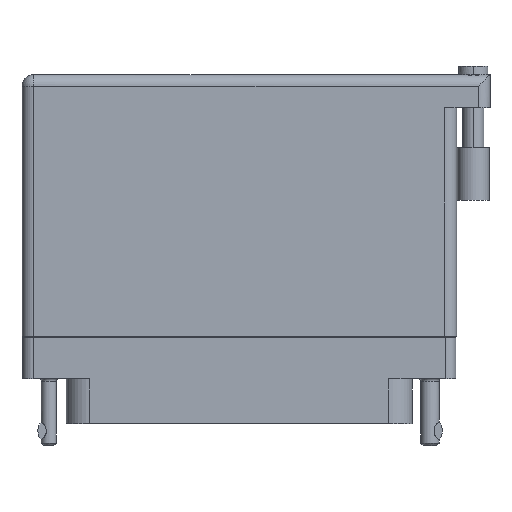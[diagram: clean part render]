
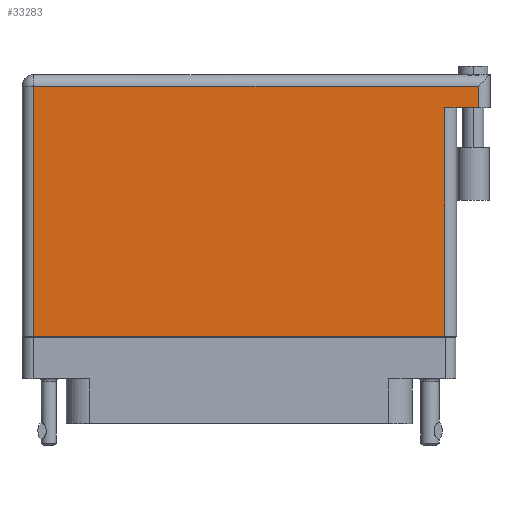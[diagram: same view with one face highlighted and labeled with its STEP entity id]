
A CAD part, front view. The second image highlights one B-rep face of the part: STEP entity #33283.
In plain terms, the highlighted face is planar.
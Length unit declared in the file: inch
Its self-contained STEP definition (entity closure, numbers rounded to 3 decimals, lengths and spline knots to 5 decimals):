
#1376 = CARTESIAN_POINT ( 'NONE',  ( 1.5, 1.269, 0.4495 ) ) ;
#2505 = LINE ( 'NONE', #43728, #18639 ) ;
#3583 = EDGE_CURVE ( 'NONE', #32225, #38675, #10501, .T. ) ;
#4847 = VECTOR ( 'NONE', #8271, 39.37008 ) ;
#5888 = ORIENTED_EDGE ( 'NONE', *, *, #9104, .T. ) ;
#6386 = CARTESIAN_POINT ( 'NONE',  ( 1.43, 1.466, 0.4495 ) ) ;
#7424 = ORIENTED_EDGE ( 'NONE', *, *, #3583, .T. ) ;
#8132 = DIRECTION ( 'NONE',  ( -1., 0., 0. ) ) ;
#8271 = DIRECTION ( 'NONE',  ( 0., -1., 0. ) ) ;
#8437 = PLANE ( 'NONE',  #33535 ) ;
#9104 = EDGE_CURVE ( 'NONE', #41778, #9441, #37307, .T. ) ;
#9441 = VERTEX_POINT ( 'NONE', #53388 ) ;
#10501 = LINE ( 'NONE', #29242, #32436 ) ;
#13491 = CARTESIAN_POINT ( 'NONE',  ( 1.23, 1.269, 0.4495 ) ) ;
#13547 = VERTEX_POINT ( 'NONE', #25972 ) ;
#13910 = CARTESIAN_POINT ( 'NONE',  ( -1.3, 1.396, 0.4495 ) ) ;
#14077 = VECTOR ( 'NONE', #29746, 39.37008 ) ;
#15924 = LINE ( 'NONE', #6386, #14077 ) ;
#18639 = VECTOR ( 'NONE', #25286, 39.37008 ) ;
#24770 = LINE ( 'NONE', #1376, #42360 ) ;
#25286 = DIRECTION ( 'NONE',  ( 1., 0., 0. ) ) ;
#25972 = CARTESIAN_POINT ( 'NONE',  ( 1.43, 1.269, 0.4495 ) ) ;
#27483 = FACE_OUTER_BOUND ( 'NONE', #33182, .T. ) ;
#29242 = CARTESIAN_POINT ( 'NONE',  ( 1.23, 1.269, 0.4495 ) ) ;
#29746 = DIRECTION ( 'NONE',  ( 0., 1., 0. ) ) ;
#30366 = CARTESIAN_POINT ( 'NONE',  ( 1.43, 1.396, 0.4495 ) ) ;
#31012 = EDGE_CURVE ( 'NONE', #9441, #52813, #31626, .T. ) ;
#31626 = LINE ( 'NONE', #50403, #4847 ) ;
#32225 = VERTEX_POINT ( 'NONE', #48055 ) ;
#32436 = VECTOR ( 'NONE', #56341, 39.37008 ) ;
#33182 = EDGE_LOOP ( 'NONE', ( #41082, #7424, #33226, #47063, #5888, #39187 ) ) ;
#33226 = ORIENTED_EDGE ( 'NONE', *, *, #40800, .F. ) ;
#33283 = ADVANCED_FACE ( 'NONE', ( #27483 ), #8437, .F. ) ;
#33535 = AXIS2_PLACEMENT_3D ( 'NONE', #36129, #54859, #8132 ) ;
#36129 = CARTESIAN_POINT ( 'NONE',  ( -1.3, 1.466, 0.4495 ) ) ;
#37307 = LINE ( 'NONE', #13910, #59516 ) ;
#38675 = VERTEX_POINT ( 'NONE', #13491 ) ;
#39187 = ORIENTED_EDGE ( 'NONE', *, *, #31012, .T. ) ;
#40800 = EDGE_CURVE ( 'NONE', #13547, #38675, #24770, .T. ) ;
#41082 = ORIENTED_EDGE ( 'NONE', *, *, #55887, .T. ) ;
#41778 = VERTEX_POINT ( 'NONE', #30366 ) ;
#42360 = VECTOR ( 'NONE', #43808, 39.37008 ) ;
#42504 = DIRECTION ( 'NONE',  ( -1., 0., 0. ) ) ;
#43728 = CARTESIAN_POINT ( 'NONE',  ( -1.3, -0.1, 0.4495 ) ) ;
#43808 = DIRECTION ( 'NONE',  ( -1., 0., 0. ) ) ;
#44584 = EDGE_CURVE ( 'NONE', #13547, #41778, #15924, .T. ) ;
#47063 = ORIENTED_EDGE ( 'NONE', *, *, #44584, .T. ) ;
#48055 = CARTESIAN_POINT ( 'NONE',  ( 1.23, -0.1, 0.4495 ) ) ;
#50403 = CARTESIAN_POINT ( 'NONE',  ( -1.23, -0.1, 0.4495 ) ) ;
#52813 = VERTEX_POINT ( 'NONE', #54882 ) ;
#53388 = CARTESIAN_POINT ( 'NONE',  ( -1.23, 1.396, 0.4495 ) ) ;
#54859 = DIRECTION ( 'NONE',  ( 0., 0., -1. ) ) ;
#54882 = CARTESIAN_POINT ( 'NONE',  ( -1.23, -0.1, 0.4495 ) ) ;
#55887 = EDGE_CURVE ( 'NONE', #52813, #32225, #2505, .T. ) ;
#56341 = DIRECTION ( 'NONE',  ( 0., 1., 0. ) ) ;
#59516 = VECTOR ( 'NONE', #42504, 39.37008 ) ;
